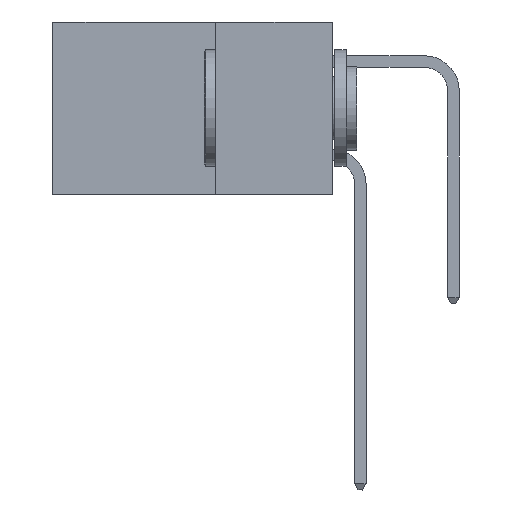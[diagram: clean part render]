
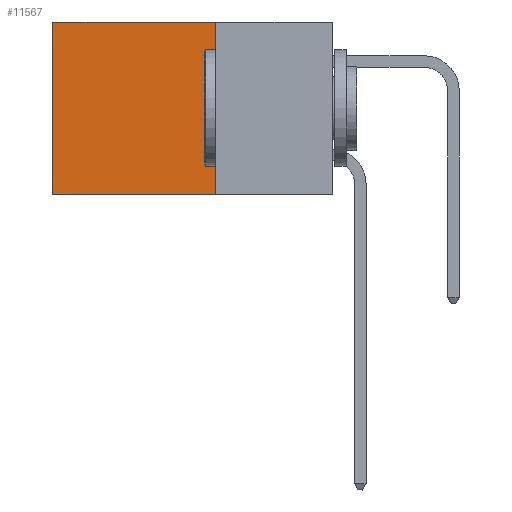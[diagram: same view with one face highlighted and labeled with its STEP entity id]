
A CAD part, left-side view. The second image highlights one B-rep face of the part: STEP entity #11567.
In plain terms, the highlighted planar face has unit normal (-1, 0, 0).
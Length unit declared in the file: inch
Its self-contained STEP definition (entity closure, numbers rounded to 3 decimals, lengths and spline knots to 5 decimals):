
#95 = CARTESIAN_POINT ( 'NONE',  ( 0.298, 0.6, 0. ) ) ;
#539 = ORIENTED_EDGE ( 'NONE', *, *, #17503, .F. ) ;
#642 = EDGE_CURVE ( 'NONE', #672, #5205, #9375, .T. ) ;
#672 = VERTEX_POINT ( 'NONE', #5956 ) ;
#3570 = CARTESIAN_POINT ( 'NONE',  ( 0.298, 0.25, 0. ) ) ;
#5205 = VERTEX_POINT ( 'NONE', #6340 ) ;
#5677 = VERTEX_POINT ( 'NONE', #8102 ) ;
#5956 = CARTESIAN_POINT ( 'NONE',  ( 0.298, 0.25, 0. ) ) ;
#6340 = CARTESIAN_POINT ( 'NONE',  ( 0.298, 0.25, -0.37 ) ) ;
#7969 = VECTOR ( 'NONE', #19469, 39.37008 ) ;
#8102 = CARTESIAN_POINT ( 'NONE',  ( 0.298, 0.6, -0.37 ) ) ;
#8904 = CARTESIAN_POINT ( 'NONE',  ( 0.298, 0.25, 0. ) ) ;
#9139 = DIRECTION ( 'NONE',  ( 0., 0., -1. ) ) ;
#9375 = LINE ( 'NONE', #14583, #7969 ) ;
#10995 = VECTOR ( 'NONE', #24099, 39.37008 ) ;
#11287 = PLANE ( 'NONE',  #15001 ) ;
#11567 = ADVANCED_FACE ( 'NONE', ( #16132 ), #11287, .F. ) ;
#11697 = LINE ( 'NONE', #28453, #10995 ) ;
#13519 = DIRECTION ( 'NONE',  ( 0., 0., -1. ) ) ;
#14583 = CARTESIAN_POINT ( 'NONE',  ( 0.298, 0.25, 0. ) ) ;
#15001 = AXIS2_PLACEMENT_3D ( 'NONE', #8904, #27027, #13519 ) ;
#15241 = VECTOR ( 'NONE', #17139, 39.37008 ) ;
#15511 = VECTOR ( 'NONE', #9139, 39.37008 ) ;
#15793 = EDGE_CURVE ( 'NONE', #23989, #5677, #27469, .T. ) ;
#16132 = FACE_OUTER_BOUND ( 'NONE', #18837, .T. ) ;
#17139 = DIRECTION ( 'NONE',  ( 0., 1., 0. ) ) ;
#17503 = EDGE_CURVE ( 'NONE', #5205, #5677, #11697, .T. ) ;
#18012 = EDGE_CURVE ( 'NONE', #672, #23989, #27202, .T. ) ;
#18073 = ORIENTED_EDGE ( 'NONE', *, *, #18012, .T. ) ;
#18837 = EDGE_LOOP ( 'NONE', ( #27680, #539, #24325, #18073 ) ) ;
#19469 = DIRECTION ( 'NONE',  ( 0., 0., -1. ) ) ;
#21425 = CARTESIAN_POINT ( 'NONE',  ( 0.298, 0.6, 0. ) ) ;
#23989 = VERTEX_POINT ( 'NONE', #21425 ) ;
#24099 = DIRECTION ( 'NONE',  ( 0., 1., 0. ) ) ;
#24325 = ORIENTED_EDGE ( 'NONE', *, *, #642, .F. ) ;
#27027 = DIRECTION ( 'NONE',  ( 1., 0., 0. ) ) ;
#27202 = LINE ( 'NONE', #3570, #15241 ) ;
#27469 = LINE ( 'NONE', #95, #15511 ) ;
#27680 = ORIENTED_EDGE ( 'NONE', *, *, #15793, .T. ) ;
#28453 = CARTESIAN_POINT ( 'NONE',  ( 0.298, 0.25, -0.37 ) ) ;
